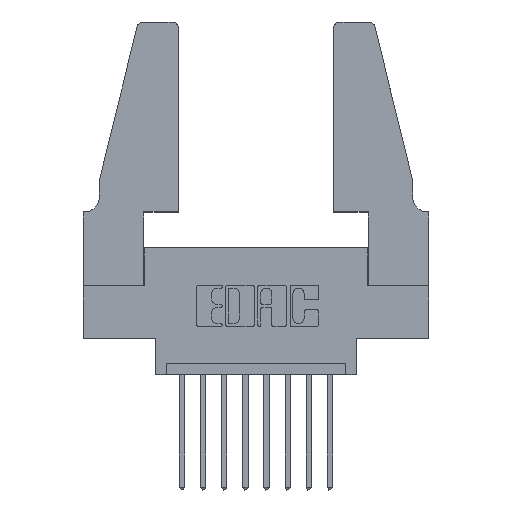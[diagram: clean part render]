
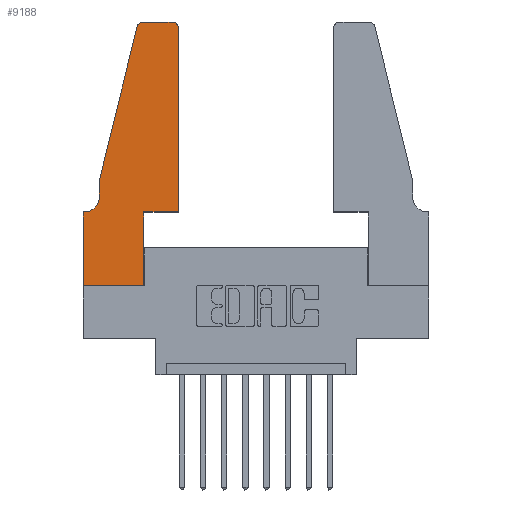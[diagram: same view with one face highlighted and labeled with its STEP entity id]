
A CAD part, top view. The second image highlights one B-rep face of the part: STEP entity #9188.
In plain terms, the highlighted planar face has unit normal (0, 0, 1).
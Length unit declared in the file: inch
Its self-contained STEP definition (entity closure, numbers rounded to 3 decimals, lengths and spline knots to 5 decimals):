
#3 = DIRECTION ( 'NONE',  ( 0., 0., 1. ) ) ;
#67 = EDGE_CURVE ( 'NONE', #11885, #10849, #3733, .T. ) ;
#187 = VERTEX_POINT ( 'NONE', #4536 ) ;
#457 = CARTESIAN_POINT ( 'NONE',  ( 0.4205, 1.25, 0.37 ) ) ;
#575 = AXIS2_PLACEMENT_3D ( 'NONE', #8576, #9374, #4406 ) ;
#578 = DIRECTION ( 'NONE',  ( 0., 0., 1. ) ) ;
#590 = PLANE ( 'NONE',  #575 ) ;
#969 = VECTOR ( 'NONE', #1549, 39.37008 ) ;
#1058 = VECTOR ( 'NONE', #3716, 39.37008 ) ;
#1217 = EDGE_CURVE ( 'NONE', #3155, #1321, #12123, .T. ) ;
#1252 = ORIENTED_EDGE ( 'NONE', *, *, #4616, .T. ) ;
#1321 = VERTEX_POINT ( 'NONE', #9848 ) ;
#1405 = VECTOR ( 'NONE', #8435, 39.37008 ) ;
#1444 = DIRECTION ( 'NONE',  ( 1., 0., 0. ) ) ;
#1507 = CARTESIAN_POINT ( 'NONE',  ( 0.4505, 0.35, 0.37 ) ) ;
#1519 = CARTESIAN_POINT ( 'NONE',  ( 0.0755, 0.5, 0.37 ) ) ;
#1549 = DIRECTION ( 'NONE',  ( 0., 1., 0. ) ) ;
#1582 = DIRECTION ( 'NONE',  ( 1., 0., 0. ) ) ;
#1794 = CIRCLE ( 'NONE', #4511, 0.03 ) ;
#2034 = CARTESIAN_POINT ( 'NONE',  ( 0., 0.35, 0.37 ) ) ;
#2150 = CARTESIAN_POINT ( 'NONE',  ( 0.25487, 1.22718, 0.37 ) ) ;
#2283 = DIRECTION ( 'NONE',  ( 0., -1., 0. ) ) ;
#2376 = DIRECTION ( 'NONE',  ( 0., 1., 0. ) ) ;
#2727 = EDGE_CURVE ( 'NONE', #12473, #11885, #11633, .T. ) ;
#2912 = VECTOR ( 'NONE', #5916, 39.37008 ) ;
#3061 = AXIS2_PLACEMENT_3D ( 'NONE', #7890, #7708, #12721 ) ;
#3155 = VERTEX_POINT ( 'NONE', #5046 ) ;
#3224 = ORIENTED_EDGE ( 'NONE', *, *, #1217, .T. ) ;
#3238 = LINE ( 'NONE', #5772, #1058 ) ;
#3258 = CARTESIAN_POINT ( 'NONE',  ( 0.0055, 0.35, 0.37 ) ) ;
#3413 = EDGE_CURVE ( 'NONE', #187, #12653, #1794, .T. ) ;
#3421 = VERTEX_POINT ( 'NONE', #8964 ) ;
#3604 = LINE ( 'NONE', #1507, #969 ) ;
#3716 = DIRECTION ( 'NONE',  ( 1., 0., 0. ) ) ;
#3733 = LINE ( 'NONE', #4346, #12471 ) ;
#4068 = DIRECTION ( 'NONE',  ( 1., 0., 0. ) ) ;
#4146 = VECTOR ( 'NONE', #1444, 39.37008 ) ;
#4346 = CARTESIAN_POINT ( 'NONE',  ( 0.0755, 0.5, 0.37 ) ) ;
#4406 = DIRECTION ( 'NONE',  ( 1., 0., 0. ) ) ;
#4511 = AXIS2_PLACEMENT_3D ( 'NONE', #11205, #578, #1582 ) ;
#4536 = CARTESIAN_POINT ( 'NONE',  ( 0.4505, 1.22, 0.37 ) ) ;
#4616 = EDGE_CURVE ( 'NONE', #10233, #3421, #10327, .T. ) ;
#4964 = CARTESIAN_POINT ( 'NONE',  ( 0.284, 1.22, 0.37 ) ) ;
#5046 = CARTESIAN_POINT ( 'NONE',  ( 0.2865, 0.35, 0.37 ) ) ;
#5715 = CIRCLE ( 'NONE', #7399, 0.03 ) ;
#5772 = CARTESIAN_POINT ( 'NONE',  ( 0., 0., 0.37 ) ) ;
#5916 = DIRECTION ( 'NONE',  ( -0.239, -0.971, 0. ) ) ;
#6154 = DIRECTION ( 'NONE',  ( -1., 0., 0. ) ) ;
#6268 = VERTEX_POINT ( 'NONE', #7378 ) ;
#6448 = EDGE_CURVE ( 'NONE', #10849, #6977, #11213, .T. ) ;
#6567 = EDGE_CURVE ( 'NONE', #12653, #8322, #6827, .T. ) ;
#6776 = ORIENTED_EDGE ( 'NONE', *, *, #10583, .T. ) ;
#6827 = LINE ( 'NONE', #11868, #11203 ) ;
#6977 = VERTEX_POINT ( 'NONE', #3258 ) ;
#7000 = CARTESIAN_POINT ( 'NONE',  ( 0.4505, 0.35, 0.37 ) ) ;
#7248 = EDGE_CURVE ( 'NONE', #6268, #3155, #7768, .T. ) ;
#7305 = EDGE_CURVE ( 'NONE', #3421, #6268, #3238, .T. ) ;
#7378 = CARTESIAN_POINT ( 'NONE',  ( 0.2865, 0., 0.37 ) ) ;
#7399 = AXIS2_PLACEMENT_3D ( 'NONE', #4964, #3, #4068 ) ;
#7624 = VECTOR ( 'NONE', #2376, 39.37008 ) ;
#7693 = VECTOR ( 'NONE', #12064, 39.37008 ) ;
#7708 = DIRECTION ( 'NONE',  ( 0., 0., -1. ) ) ;
#7768 = LINE ( 'NONE', #9414, #7624 ) ;
#7890 = CARTESIAN_POINT ( 'NONE',  ( 0.0055, 0.42, 0.37 ) ) ;
#8004 = ORIENTED_EDGE ( 'NONE', *, *, #2727, .T. ) ;
#8149 = ORIENTED_EDGE ( 'NONE', *, *, #67, .T. ) ;
#8322 = VERTEX_POINT ( 'NONE', #8509 ) ;
#8333 = EDGE_CURVE ( 'NONE', #8322, #12473, #5715, .T. ) ;
#8435 = DIRECTION ( 'NONE',  ( -1., 0., 0. ) ) ;
#8509 = CARTESIAN_POINT ( 'NONE',  ( 0.284, 1.25, 0.37 ) ) ;
#8576 = CARTESIAN_POINT ( 'NONE',  ( 0., 0.35, 0.37 ) ) ;
#8964 = CARTESIAN_POINT ( 'NONE',  ( 0., 0., 0.37 ) ) ;
#9152 = EDGE_CURVE ( 'NONE', #1321, #187, #3604, .T. ) ;
#9188 = ADVANCED_FACE ( 'NONE', ( #10721 ), #590, .T. ) ;
#9306 = CARTESIAN_POINT ( 'NONE',  ( 0., 0., 0.37 ) ) ;
#9374 = DIRECTION ( 'NONE',  ( 0., 0., 1. ) ) ;
#9414 = CARTESIAN_POINT ( 'NONE',  ( 0.2865, 0.35, 0.37 ) ) ;
#9848 = CARTESIAN_POINT ( 'NONE',  ( 0.4505, 0.35, 0.37 ) ) ;
#10233 = VERTEX_POINT ( 'NONE', #2034 ) ;
#10327 = LINE ( 'NONE', #9306, #7693 ) ;
#10356 = EDGE_LOOP ( 'NONE', ( #11416, #11536, #8004, #8149, #11571, #6776, #1252, #11767, #12030, #3224, #10430, #12679 ) ) ;
#10430 = ORIENTED_EDGE ( 'NONE', *, *, #9152, .T. ) ;
#10583 = EDGE_CURVE ( 'NONE', #6977, #10233, #11065, .T. ) ;
#10600 = CARTESIAN_POINT ( 'NONE',  ( 0.0755, 0.42, 0.37 ) ) ;
#10721 = FACE_OUTER_BOUND ( 'NONE', #10356, .T. ) ;
#10849 = VERTEX_POINT ( 'NONE', #10600 ) ;
#11065 = LINE ( 'NONE', #11117, #1405 ) ;
#11117 = CARTESIAN_POINT ( 'NONE',  ( 0.0755, 0.35, 0.37 ) ) ;
#11203 = VECTOR ( 'NONE', #6154, 39.37008 ) ;
#11205 = CARTESIAN_POINT ( 'NONE',  ( 0.4205, 1.22, 0.37 ) ) ;
#11213 = CIRCLE ( 'NONE', #3061, 0.07 ) ;
#11416 = ORIENTED_EDGE ( 'NONE', *, *, #6567, .T. ) ;
#11536 = ORIENTED_EDGE ( 'NONE', *, *, #8333, .T. ) ;
#11571 = ORIENTED_EDGE ( 'NONE', *, *, #6448, .T. ) ;
#11633 = LINE ( 'NONE', #11871, #2912 ) ;
#11767 = ORIENTED_EDGE ( 'NONE', *, *, #7305, .T. ) ;
#11868 = CARTESIAN_POINT ( 'NONE',  ( 0.2605, 1.25, 0.37 ) ) ;
#11871 = CARTESIAN_POINT ( 'NONE',  ( 0.0755, 0.5, 0.37 ) ) ;
#11885 = VERTEX_POINT ( 'NONE', #1519 ) ;
#12030 = ORIENTED_EDGE ( 'NONE', *, *, #7248, .T. ) ;
#12064 = DIRECTION ( 'NONE',  ( 0., -1., 0. ) ) ;
#12123 = LINE ( 'NONE', #7000, #4146 ) ;
#12471 = VECTOR ( 'NONE', #2283, 39.37008 ) ;
#12473 = VERTEX_POINT ( 'NONE', #2150 ) ;
#12653 = VERTEX_POINT ( 'NONE', #457 ) ;
#12679 = ORIENTED_EDGE ( 'NONE', *, *, #3413, .T. ) ;
#12721 = DIRECTION ( 'NONE',  ( -1., 0., 0. ) ) ;
